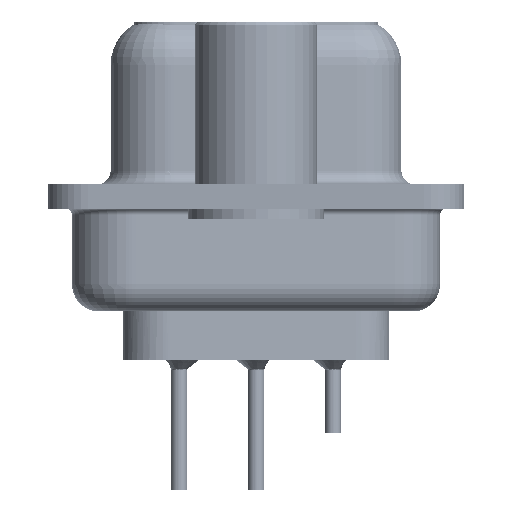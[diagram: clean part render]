
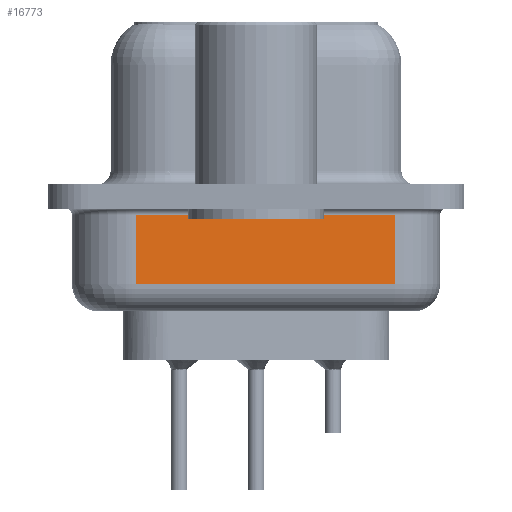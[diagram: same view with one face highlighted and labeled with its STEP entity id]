
A CAD part, left-side view. The second image highlights one B-rep face of the part: STEP entity #16773.
In plain terms, the highlighted planar face has unit normal (-0.985, -0.174, 0).
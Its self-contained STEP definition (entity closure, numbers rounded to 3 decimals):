
#2040 = CARTESIAN_POINT ( 'NONE',  ( 4.623, -5.147, -4.25 ) ) ;
#2641 = VERTEX_POINT ( 'NONE', #38535 ) ;
#3851 = EDGE_CURVE ( 'NONE', #39764, #41372, #35293, .T. ) ;
#10111 = DIRECTION ( 'NONE',  ( -0.174, 0.985, 0. ) ) ;
#10145 = CARTESIAN_POINT ( 'NONE',  ( 2.93, 4.453, -4.25 ) ) ;
#11028 = DIRECTION ( 'NONE',  ( 0.174, -0.985, 0. ) ) ;
#13238 = DIRECTION ( 'NONE',  ( -0.174, 0.985, 0. ) ) ;
#14482 = DIRECTION ( 'NONE',  ( 0., 0., 1. ) ) ;
#16093 = PLANE ( 'NONE',  #24495 ) ;
#16773 = ADVANCED_FACE ( 'NONE', ( #23724 ), #16093, .F. ) ;
#16967 = VECTOR ( 'NONE', #28697, 1000. ) ;
#17148 = EDGE_CURVE ( 'NONE', #39764, #2641, #40056, .T. ) ;
#18494 = CARTESIAN_POINT ( 'NONE',  ( 4.623, -5.147, -0.7 ) ) ;
#18597 = EDGE_CURVE ( 'NONE', #41372, #40009, #34826, .T. ) ;
#19036 = VECTOR ( 'NONE', #10111, 1000. ) ;
#19936 = EDGE_CURVE ( 'NONE', #40009, #2641, #26486, .T. ) ;
#20322 = VECTOR ( 'NONE', #14482, 1000. ) ;
#21736 = ORIENTED_EDGE ( 'NONE', *, *, #19936, .T. ) ;
#23724 = FACE_OUTER_BOUND ( 'NONE', #25650, .T. ) ;
#24495 = AXIS2_PLACEMENT_3D ( 'NONE', #37061, #43188, #13238 ) ;
#24999 = CARTESIAN_POINT ( 'NONE',  ( 2.93, 4.453, -3.25 ) ) ;
#25650 = EDGE_LOOP ( 'NONE', ( #33861, #34358, #33500, #21736 ) ) ;
#26486 = LINE ( 'NONE', #43106, #19036 ) ;
#28697 = DIRECTION ( 'NONE',  ( 0., 0., 1. ) ) ;
#33500 = ORIENTED_EDGE ( 'NONE', *, *, #18597, .T. ) ;
#33861 = ORIENTED_EDGE ( 'NONE', *, *, #17148, .F. ) ;
#34358 = ORIENTED_EDGE ( 'NONE', *, *, #3851, .T. ) ;
#34826 = LINE ( 'NONE', #2040, #16967 ) ;
#35293 = LINE ( 'NONE', #24999, #38765 ) ;
#36017 = CARTESIAN_POINT ( 'NONE',  ( 4.623, -5.147, -3.25 ) ) ;
#37061 = CARTESIAN_POINT ( 'NONE',  ( 2.93, 4.453, -4.25 ) ) ;
#38535 = CARTESIAN_POINT ( 'NONE',  ( 2.93, 4.453, -0.7 ) ) ;
#38765 = VECTOR ( 'NONE', #11028, 1000. ) ;
#39764 = VERTEX_POINT ( 'NONE', #43033 ) ;
#40009 = VERTEX_POINT ( 'NONE', #18494 ) ;
#40056 = LINE ( 'NONE', #10145, #20322 ) ;
#41372 = VERTEX_POINT ( 'NONE', #36017 ) ;
#43033 = CARTESIAN_POINT ( 'NONE',  ( 2.93, 4.453, -3.25 ) ) ;
#43106 = CARTESIAN_POINT ( 'NONE',  ( 2.93, 4.453, -0.7 ) ) ;
#43188 = DIRECTION ( 'NONE',  ( 0.985, 0.174, 0. ) ) ;
